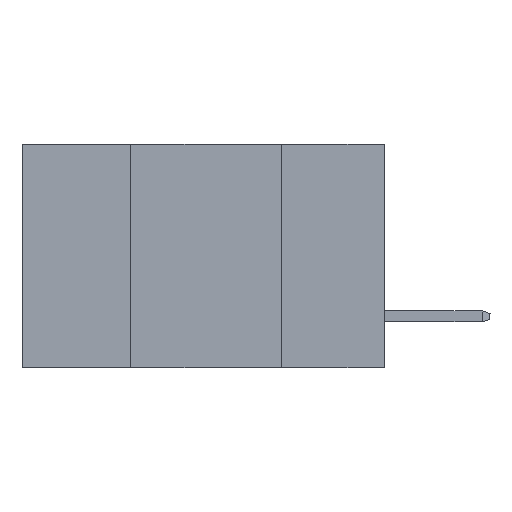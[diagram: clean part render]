
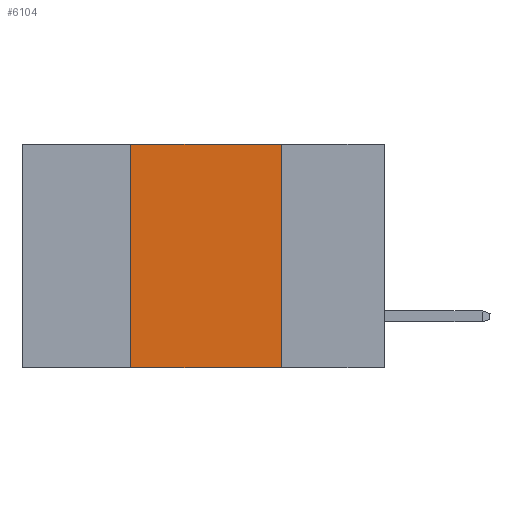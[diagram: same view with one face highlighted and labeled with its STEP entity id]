
A CAD part, left-side view. The second image highlights one B-rep face of the part: STEP entity #6104.
In plain terms, the highlighted planar face has unit normal (-1, 0, 0).
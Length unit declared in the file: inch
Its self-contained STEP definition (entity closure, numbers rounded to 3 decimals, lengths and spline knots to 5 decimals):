
#1322 = CARTESIAN_POINT ( 'NONE',  ( 0., 0.6, -0.37 ) ) ;
#1353 = VERTEX_POINT ( 'NONE', #7680 ) ;
#1487 = ORIENTED_EDGE ( 'NONE', *, *, #19650, .F. ) ;
#4791 = DIRECTION ( 'NONE',  ( 0., 0., 1. ) ) ;
#5735 = CARTESIAN_POINT ( 'NONE',  ( 0., 0.17, -0.37 ) ) ;
#6104 = ADVANCED_FACE ( 'NONE', ( #12144 ), #16889, .F. ) ;
#7486 = EDGE_CURVE ( 'NONE', #15073, #21583, #20045, .T. ) ;
#7680 = CARTESIAN_POINT ( 'NONE',  ( 0., 0.42, 0. ) ) ;
#7980 = LINE ( 'NONE', #23669, #12550 ) ;
#8356 = CARTESIAN_POINT ( 'NONE',  ( 0., 0.42, 0. ) ) ;
#10737 = EDGE_CURVE ( 'NONE', #1353, #14065, #7980, .T. ) ;
#11060 = LINE ( 'NONE', #8356, #18706 ) ;
#11409 = VECTOR ( 'NONE', #12425, 39.37008 ) ;
#11527 = CARTESIAN_POINT ( 'NONE',  ( 0., 0.42, -0.37 ) ) ;
#12144 = FACE_OUTER_BOUND ( 'NONE', #22707, .T. ) ;
#12425 = DIRECTION ( 'NONE',  ( 0., 0., -1. ) ) ;
#12550 = VECTOR ( 'NONE', #20223, 39.37008 ) ;
#13060 = CARTESIAN_POINT ( 'NONE',  ( 0., 0.6, 0. ) ) ;
#14065 = VERTEX_POINT ( 'NONE', #14981 ) ;
#14946 = ORIENTED_EDGE ( 'NONE', *, *, #10737, .F. ) ;
#14981 = CARTESIAN_POINT ( 'NONE',  ( 0., 0.17, 0. ) ) ;
#15012 = DIRECTION ( 'NONE',  ( 0., 0., -1. ) ) ;
#15073 = VERTEX_POINT ( 'NONE', #11527 ) ;
#16626 = EDGE_CURVE ( 'NONE', #15073, #1353, #11060, .T. ) ;
#16889 = PLANE ( 'NONE',  #18179 ) ;
#17872 = LINE ( 'NONE', #24130, #11409 ) ;
#18179 = AXIS2_PLACEMENT_3D ( 'NONE', #13060, #20798, #15012 ) ;
#18640 = DIRECTION ( 'NONE',  ( 0., -1., 0. ) ) ;
#18706 = VECTOR ( 'NONE', #4791, 39.37008 ) ;
#19650 = EDGE_CURVE ( 'NONE', #14065, #21583, #17872, .T. ) ;
#20045 = LINE ( 'NONE', #1322, #20613 ) ;
#20223 = DIRECTION ( 'NONE',  ( 0., -1., 0. ) ) ;
#20613 = VECTOR ( 'NONE', #18640, 39.37008 ) ;
#20798 = DIRECTION ( 'NONE',  ( 1., 0., 0. ) ) ;
#21583 = VERTEX_POINT ( 'NONE', #5735 ) ;
#22646 = ORIENTED_EDGE ( 'NONE', *, *, #7486, .T. ) ;
#22707 = EDGE_LOOP ( 'NONE', ( #1487, #14946, #25095, #22646 ) ) ;
#23669 = CARTESIAN_POINT ( 'NONE',  ( 0., 0.6, 0. ) ) ;
#24130 = CARTESIAN_POINT ( 'NONE',  ( 0., 0.17, 0. ) ) ;
#25095 = ORIENTED_EDGE ( 'NONE', *, *, #16626, .F. ) ;
